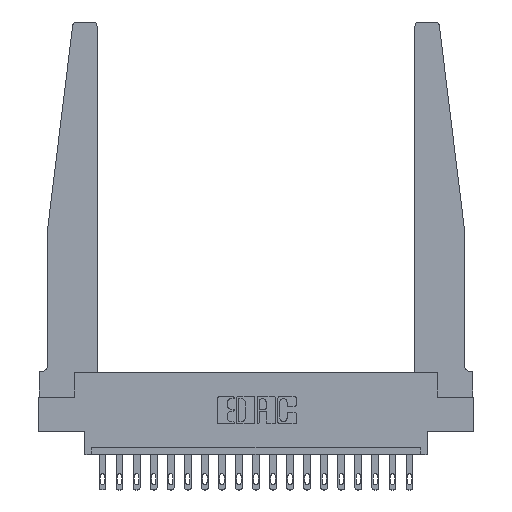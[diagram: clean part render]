
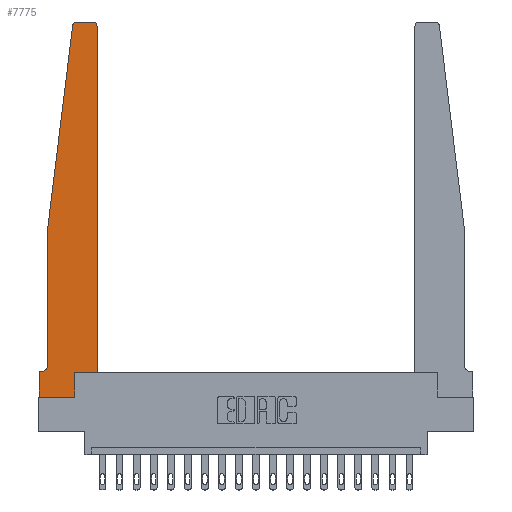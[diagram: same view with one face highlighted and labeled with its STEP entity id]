
A CAD part, top view. The second image highlights one B-rep face of the part: STEP entity #7775.
In plain terms, the highlighted planar face has unit normal (0, 0, 1).
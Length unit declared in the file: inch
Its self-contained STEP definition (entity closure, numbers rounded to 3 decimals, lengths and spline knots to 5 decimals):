
#188 = PLANE ( 'NONE',  #19345 ) ;
#232 = VERTEX_POINT ( 'NONE', #5770 ) ;
#283 = CARTESIAN_POINT ( 'NONE',  ( 0., 0.1875, 0.37 ) ) ;
#287 = CARTESIAN_POINT ( 'NONE',  ( 0.2605, 0.18, 0.37 ) ) ;
#491 = ORIENTED_EDGE ( 'NONE', *, *, #2734, .T. ) ;
#623 = DIRECTION ( 'NONE',  ( -1., 0., 0. ) ) ;
#921 = CARTESIAN_POINT ( 'NONE',  ( 0.395, 2.72, 0.37 ) ) ;
#938 = CIRCLE ( 'NONE', #10396, 0.03 ) ;
#1058 = ORIENTED_EDGE ( 'NONE', *, *, #11121, .T. ) ;
#1269 = DIRECTION ( 'NONE',  ( 1., 0., 0. ) ) ;
#1431 = VECTOR ( 'NONE', #6879, 39.37008 ) ;
#1791 = DIRECTION ( 'NONE',  ( 1., 0., 0. ) ) ;
#2734 = EDGE_CURVE ( 'NONE', #4572, #17507, #14450, .T. ) ;
#2765 = CARTESIAN_POINT ( 'NONE',  ( 0.065, 1.25, 0.37 ) ) ;
#3029 = ORIENTED_EDGE ( 'NONE', *, *, #5009, .T. ) ;
#3280 = DIRECTION ( 'NONE',  ( 0., 1., 0. ) ) ;
#3339 = CIRCLE ( 'NONE', #4683, 0.05 ) ;
#3619 = VERTEX_POINT ( 'NONE', #17036 ) ;
#3815 = LINE ( 'NONE', #8494, #1431 ) ;
#4003 = DIRECTION ( 'NONE',  ( 0., -1., 0. ) ) ;
#4572 = VERTEX_POINT ( 'NONE', #16235 ) ;
#4599 = DIRECTION ( 'NONE',  ( 0., 0., 1. ) ) ;
#4683 = AXIS2_PLACEMENT_3D ( 'NONE', #5290, #6618, #5096 ) ;
#4703 = DIRECTION ( 'NONE',  ( 0., -1., 0. ) ) ;
#5009 = EDGE_CURVE ( 'NONE', #11414, #18836, #3339, .T. ) ;
#5096 = DIRECTION ( 'NONE',  ( -1., 0., 0. ) ) ;
#5189 = CARTESIAN_POINT ( 'NONE',  ( 0.065, 0.1875, 0.37 ) ) ;
#5287 = LINE ( 'NONE', #5189, #6171 ) ;
#5290 = CARTESIAN_POINT ( 'NONE',  ( 0.015, 0.2375, 0.37 ) ) ;
#5336 = CARTESIAN_POINT ( 'NONE',  ( 0.065, 1.25, 0.37 ) ) ;
#5346 = ORIENTED_EDGE ( 'NONE', *, *, #5755, .T. ) ;
#5394 = VECTOR ( 'NONE', #1269, 39.37008 ) ;
#5578 = ORIENTED_EDGE ( 'NONE', *, *, #6118, .T. ) ;
#5623 = DIRECTION ( 'NONE',  ( 0., 0., 1. ) ) ;
#5742 = CARTESIAN_POINT ( 'NONE',  ( 0.065, 1.25, 0.37 ) ) ;
#5755 = EDGE_CURVE ( 'NONE', #13501, #4572, #12098, .T. ) ;
#5770 = CARTESIAN_POINT ( 'NONE',  ( 0., 0.1875, 0.37 ) ) ;
#6118 = EDGE_CURVE ( 'NONE', #232, #13501, #7660, .T. ) ;
#6154 = VECTOR ( 'NONE', #3280, 39.37008 ) ;
#6171 = VECTOR ( 'NONE', #17408, 39.37008 ) ;
#6473 = VECTOR ( 'NONE', #623, 39.37008 ) ;
#6618 = DIRECTION ( 'NONE',  ( 0., 0., -1. ) ) ;
#6720 = DIRECTION ( 'NONE',  ( 0., 1., 0. ) ) ;
#6777 = LINE ( 'NONE', #5336, #12939 ) ;
#6879 = DIRECTION ( 'NONE',  ( 1., 0., 0. ) ) ;
#7564 = EDGE_CURVE ( 'NONE', #9873, #11124, #19071, .T. ) ;
#7660 = LINE ( 'NONE', #18468, #10954 ) ;
#7775 = ADVANCED_FACE ( 'NONE', ( #12932 ), #188, .T. ) ;
#8382 = LINE ( 'NONE', #14599, #6473 ) ;
#8494 = CARTESIAN_POINT ( 'NONE',  ( 0.425, 0.18, 0.37 ) ) ;
#8990 = DIRECTION ( 'NONE',  ( 1., 0., 0. ) ) ;
#9873 = VERTEX_POINT ( 'NONE', #18791 ) ;
#10193 = CARTESIAN_POINT ( 'NONE',  ( 0.015, 0.1875, 0.37 ) ) ;
#10396 = AXIS2_PLACEMENT_3D ( 'NONE', #18641, #4599, #10801 ) ;
#10801 = DIRECTION ( 'NONE',  ( 1., 0., 0. ) ) ;
#10883 = CARTESIAN_POINT ( 'NONE',  ( 0.2605, 0.18, 0.37 ) ) ;
#10954 = VECTOR ( 'NONE', #4703, 39.37008 ) ;
#11121 = EDGE_CURVE ( 'NONE', #11170, #11414, #17964, .T. ) ;
#11124 = VERTEX_POINT ( 'NONE', #12062 ) ;
#11170 = VERTEX_POINT ( 'NONE', #2765 ) ;
#11336 = CARTESIAN_POINT ( 'NONE',  ( 0.425, 0.18, 0.37 ) ) ;
#11414 = VERTEX_POINT ( 'NONE', #17726 ) ;
#12062 = CARTESIAN_POINT ( 'NONE',  ( 0.425, 2.72, 0.37 ) ) ;
#12098 = LINE ( 'NONE', #16698, #5394 ) ;
#12252 = ORIENTED_EDGE ( 'NONE', *, *, #19250, .T. ) ;
#12932 = FACE_OUTER_BOUND ( 'NONE', #19130, .T. ) ;
#12939 = VECTOR ( 'NONE', #19508, 39.37008 ) ;
#13419 = EDGE_CURVE ( 'NONE', #17507, #9873, #3815, .T. ) ;
#13501 = VERTEX_POINT ( 'NONE', #15958 ) ;
#14316 = VECTOR ( 'NONE', #6720, 39.37008 ) ;
#14450 = LINE ( 'NONE', #287, #14316 ) ;
#14599 = CARTESIAN_POINT ( 'NONE',  ( 0.25, 2.75, 0.37 ) ) ;
#14793 = CIRCLE ( 'NONE', #19359, 0.03 ) ;
#14820 = VERTEX_POINT ( 'NONE', #19721 ) ;
#15098 = ORIENTED_EDGE ( 'NONE', *, *, #7564, .T. ) ;
#15213 = EDGE_CURVE ( 'NONE', #11124, #14820, #14793, .T. ) ;
#15218 = ORIENTED_EDGE ( 'NONE', *, *, #19986, .T. ) ;
#15708 = DIRECTION ( 'NONE',  ( 0., 0., 1. ) ) ;
#15958 = CARTESIAN_POINT ( 'NONE',  ( 0., 0., 0.37 ) ) ;
#16174 = VERTEX_POINT ( 'NONE', #17513 ) ;
#16235 = CARTESIAN_POINT ( 'NONE',  ( 0.2605, 0., 0.37 ) ) ;
#16698 = CARTESIAN_POINT ( 'NONE',  ( 0., 0., 0.37 ) ) ;
#17036 = CARTESIAN_POINT ( 'NONE',  ( 0.27653, 2.75, 0.37 ) ) ;
#17402 = VECTOR ( 'NONE', #4003, 39.37008 ) ;
#17408 = DIRECTION ( 'NONE',  ( -1., 0., 0. ) ) ;
#17507 = VERTEX_POINT ( 'NONE', #10883 ) ;
#17513 = CARTESIAN_POINT ( 'NONE',  ( 0.24675, 2.72367, 0.37 ) ) ;
#17629 = ORIENTED_EDGE ( 'NONE', *, *, #15213, .T. ) ;
#17726 = CARTESIAN_POINT ( 'NONE',  ( 0.065, 0.2375, 0.37 ) ) ;
#17964 = LINE ( 'NONE', #5742, #17402 ) ;
#18149 = EDGE_CURVE ( 'NONE', #16174, #11170, #6777, .T. ) ;
#18468 = CARTESIAN_POINT ( 'NONE',  ( 0., 0., 0.37 ) ) ;
#18641 = CARTESIAN_POINT ( 'NONE',  ( 0.27653, 2.72, 0.37 ) ) ;
#18791 = CARTESIAN_POINT ( 'NONE',  ( 0.425, 0.18, 0.37 ) ) ;
#18836 = VERTEX_POINT ( 'NONE', #10193 ) ;
#18861 = ORIENTED_EDGE ( 'NONE', *, *, #13419, .T. ) ;
#19071 = LINE ( 'NONE', #11336, #6154 ) ;
#19130 = EDGE_LOOP ( 'NONE', ( #12252, #19682, #19932, #1058, #3029, #15218, #5578, #5346, #491, #18861, #15098, #17629 ) ) ;
#19250 = EDGE_CURVE ( 'NONE', #14820, #3619, #8382, .T. ) ;
#19345 = AXIS2_PLACEMENT_3D ( 'NONE', #283, #15708, #1791 ) ;
#19359 = AXIS2_PLACEMENT_3D ( 'NONE', #921, #5623, #8990 ) ;
#19508 = DIRECTION ( 'NONE',  ( -0.122, -0.992, 0. ) ) ;
#19682 = ORIENTED_EDGE ( 'NONE', *, *, #19743, .T. ) ;
#19721 = CARTESIAN_POINT ( 'NONE',  ( 0.395, 2.75, 0.37 ) ) ;
#19743 = EDGE_CURVE ( 'NONE', #3619, #16174, #938, .T. ) ;
#19932 = ORIENTED_EDGE ( 'NONE', *, *, #18149, .T. ) ;
#19986 = EDGE_CURVE ( 'NONE', #18836, #232, #5287, .T. ) ;
